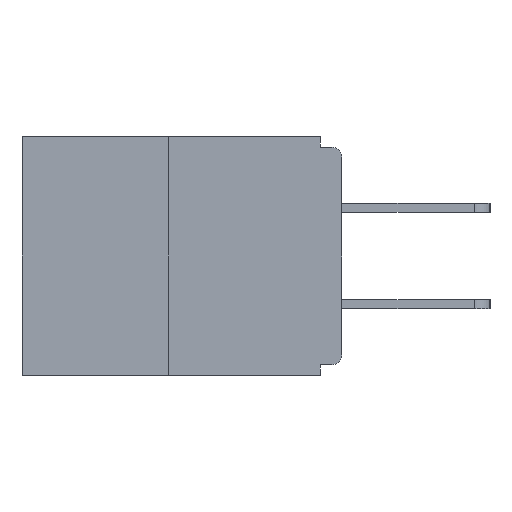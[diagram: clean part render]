
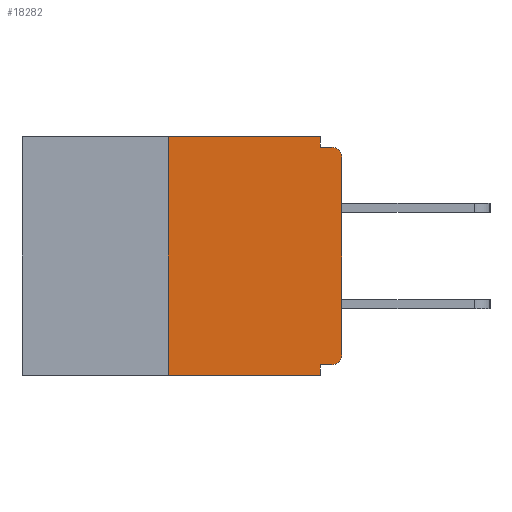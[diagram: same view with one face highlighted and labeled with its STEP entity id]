
A CAD part, left-side view. The second image highlights one B-rep face of the part: STEP entity #18282.
In plain terms, the highlighted planar face has unit normal (-1, 0, 0).
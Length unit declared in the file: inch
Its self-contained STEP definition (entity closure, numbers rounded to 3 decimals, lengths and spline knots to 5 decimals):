
#164 = LINE ( 'NONE', #20073, #20272 ) ;
#202 = LINE ( 'NONE', #8733, #13376 ) ;
#269 = EDGE_CURVE ( 'NONE', #11986, #16142, #24315, .T. ) ;
#1663 = LINE ( 'NONE', #6261, #11800 ) ;
#2104 = EDGE_CURVE ( 'NONE', #8753, #22334, #26081, .T. ) ;
#3264 = CARTESIAN_POINT ( 'NONE',  ( 0., 0., 0. ) ) ;
#3503 = DIRECTION ( 'NONE',  ( 0., 0., -1. ) ) ;
#3880 = DIRECTION ( 'NONE',  ( 0., 0., -1. ) ) ;
#4524 = CARTESIAN_POINT ( 'NONE',  ( 0., 0.015, -0.328 ) ) ;
#4731 = ORIENTED_EDGE ( 'NONE', *, *, #19675, .F. ) ;
#4735 = VERTEX_POINT ( 'NONE', #8271 ) ;
#4777 = EDGE_CURVE ( 'NONE', #11922, #16142, #1663, .T. ) ;
#5409 = ORIENTED_EDGE ( 'NONE', *, *, #13776, .F. ) ;
#5660 = DIRECTION ( 'NONE',  ( -1., 0., 0. ) ) ;
#5684 = CARTESIAN_POINT ( 'NONE',  ( 0., 0.46, 0. ) ) ;
#6027 = CARTESIAN_POINT ( 'NONE',  ( 0., 0.015, -0.313 ) ) ;
#6213 = CARTESIAN_POINT ( 'NONE',  ( 0., 0.031, 0. ) ) ;
#6261 = CARTESIAN_POINT ( 'NONE',  ( 0., 0.031, -0.343 ) ) ;
#7427 = DIRECTION ( 'NONE',  ( 0., 0., 1. ) ) ;
#8271 = CARTESIAN_POINT ( 'NONE',  ( 0., 0.031, -0.015 ) ) ;
#8326 = ORIENTED_EDGE ( 'NONE', *, *, #2104, .T. ) ;
#8549 = DIRECTION ( 'NONE',  ( 0., 1., 0. ) ) ;
#8733 = CARTESIAN_POINT ( 'NONE',  ( 0., 0., -0.015 ) ) ;
#8753 = VERTEX_POINT ( 'NONE', #20388 ) ;
#8999 = DIRECTION ( 'NONE',  ( 0., -1., 0. ) ) ;
#9391 = ORIENTED_EDGE ( 'NONE', *, *, #22606, .F. ) ;
#9430 = DIRECTION ( 'NONE',  ( 0., 0., 1. ) ) ;
#10298 = DIRECTION ( 'NONE',  ( 0., -1., 0. ) ) ;
#10617 = CIRCLE ( 'NONE', #13806, 0.015 ) ;
#11435 = VERTEX_POINT ( 'NONE', #24898 ) ;
#11649 = AXIS2_PLACEMENT_3D ( 'NONE', #27852, #12150, #20935 ) ;
#11755 = CARTESIAN_POINT ( 'NONE',  ( 0., 0.031, -0.328 ) ) ;
#11800 = VECTOR ( 'NONE', #14789, 39.37008 ) ;
#11888 = CARTESIAN_POINT ( 'NONE',  ( 0., 0.25, 0. ) ) ;
#11892 = LINE ( 'NONE', #3264, #19666 ) ;
#11922 = VERTEX_POINT ( 'NONE', #11755 ) ;
#11986 = VERTEX_POINT ( 'NONE', #16391 ) ;
#12150 = DIRECTION ( 'NONE',  ( 1., 0., 0. ) ) ;
#12290 = PLANE ( 'NONE',  #11649 ) ;
#13100 = DIRECTION ( 'NONE',  ( 0., -1., 0. ) ) ;
#13233 = CARTESIAN_POINT ( 'NONE',  ( 0., 0.46, -0.343 ) ) ;
#13376 = VECTOR ( 'NONE', #8999, 39.37008 ) ;
#13776 = EDGE_CURVE ( 'NONE', #4735, #22334, #202, .T. ) ;
#13806 = AXIS2_PLACEMENT_3D ( 'NONE', #6027, #26169, #3880 ) ;
#14205 = VECTOR ( 'NONE', #13100, 39.37008 ) ;
#14761 = ORIENTED_EDGE ( 'NONE', *, *, #269, .T. ) ;
#14789 = DIRECTION ( 'NONE',  ( 0., 0., -1. ) ) ;
#15005 = DIRECTION ( 'NONE',  ( 0., 0., -1. ) ) ;
#15807 = ORIENTED_EDGE ( 'NONE', *, *, #24664, .T. ) ;
#15875 = CARTESIAN_POINT ( 'NONE',  ( 0., 0.015, -0.015 ) ) ;
#16142 = VERTEX_POINT ( 'NONE', #20554 ) ;
#16188 = VECTOR ( 'NONE', #9430, 39.37008 ) ;
#16391 = CARTESIAN_POINT ( 'NONE',  ( 0., 0.25, -0.343 ) ) ;
#16934 = ORIENTED_EDGE ( 'NONE', *, *, #27126, .F. ) ;
#18063 = ORIENTED_EDGE ( 'NONE', *, *, #23071, .T. ) ;
#18282 = ADVANCED_FACE ( 'NONE', ( #18631 ), #12290, .F. ) ;
#18631 = FACE_OUTER_BOUND ( 'NONE', #18663, .T. ) ;
#18663 = EDGE_LOOP ( 'NONE', ( #4731, #16934, #14761, #24371, #24550, #18063, #15807, #8326, #5409, #9391 ) ) ;
#19604 = LINE ( 'NONE', #6213, #26206 ) ;
#19666 = VECTOR ( 'NONE', #7427, 39.37008 ) ;
#19675 = EDGE_CURVE ( 'NONE', #25960, #19959, #25414, .T. ) ;
#19959 = VERTEX_POINT ( 'NONE', #23064 ) ;
#20073 = CARTESIAN_POINT ( 'NONE',  ( 0., 0., -0.328 ) ) ;
#20272 = VECTOR ( 'NONE', #8549, 39.37008 ) ;
#20388 = CARTESIAN_POINT ( 'NONE',  ( 0., 0., -0.03 ) ) ;
#20554 = CARTESIAN_POINT ( 'NONE',  ( 0., 0.031, -0.343 ) ) ;
#20935 = DIRECTION ( 'NONE',  ( 0., 0., -1. ) ) ;
#21952 = CARTESIAN_POINT ( 'NONE',  ( 0., 0.25, 0. ) ) ;
#22334 = VERTEX_POINT ( 'NONE', #15875 ) ;
#22538 = LINE ( 'NONE', #11888, #16188 ) ;
#22606 = EDGE_CURVE ( 'NONE', #19959, #4735, #19604, .T. ) ;
#22842 = AXIS2_PLACEMENT_3D ( 'NONE', #25674, #5660, #3503 ) ;
#22929 = VECTOR ( 'NONE', #10298, 39.37008 ) ;
#23064 = CARTESIAN_POINT ( 'NONE',  ( 0., 0.031, 0. ) ) ;
#23071 = EDGE_CURVE ( 'NONE', #24981, #11435, #10617, .T. ) ;
#23640 = EDGE_CURVE ( 'NONE', #24981, #11922, #164, .T. ) ;
#24315 = LINE ( 'NONE', #13233, #14205 ) ;
#24371 = ORIENTED_EDGE ( 'NONE', *, *, #4777, .F. ) ;
#24550 = ORIENTED_EDGE ( 'NONE', *, *, #23640, .F. ) ;
#24664 = EDGE_CURVE ( 'NONE', #11435, #8753, #11892, .T. ) ;
#24898 = CARTESIAN_POINT ( 'NONE',  ( 0., 0., -0.313 ) ) ;
#24981 = VERTEX_POINT ( 'NONE', #4524 ) ;
#25414 = LINE ( 'NONE', #5684, #22929 ) ;
#25674 = CARTESIAN_POINT ( 'NONE',  ( 0., 0.015, -0.03 ) ) ;
#25960 = VERTEX_POINT ( 'NONE', #21952 ) ;
#26081 = CIRCLE ( 'NONE', #22842, 0.015 ) ;
#26169 = DIRECTION ( 'NONE',  ( -1., 0., 0. ) ) ;
#26206 = VECTOR ( 'NONE', #15005, 39.37008 ) ;
#27126 = EDGE_CURVE ( 'NONE', #11986, #25960, #22538, .T. ) ;
#27852 = CARTESIAN_POINT ( 'NONE',  ( 0., 0.46, 0. ) ) ;
